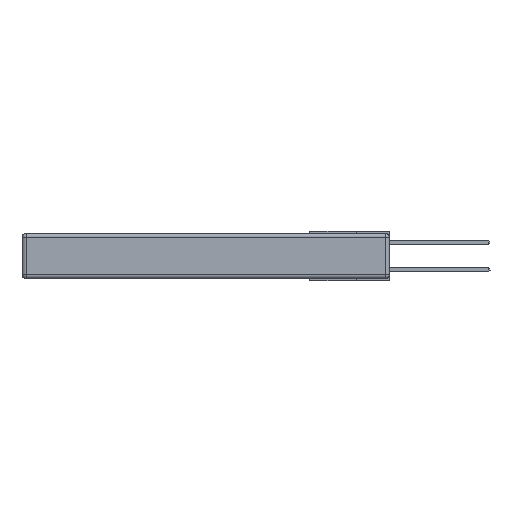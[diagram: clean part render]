
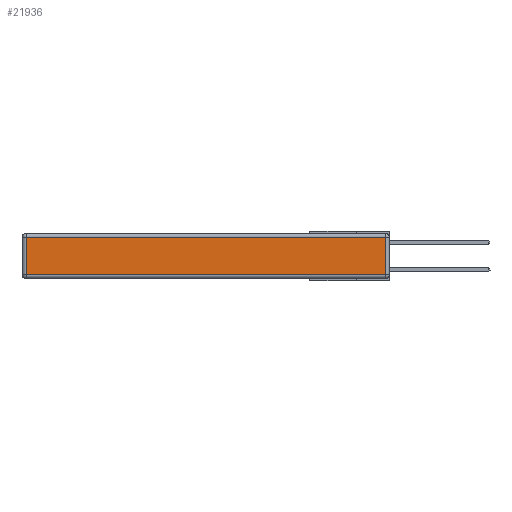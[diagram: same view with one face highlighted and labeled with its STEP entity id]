
A CAD part, left-side view. The second image highlights one B-rep face of the part: STEP entity #21936.
In plain terms, the highlighted planar face has unit normal (-1, 0, 0).
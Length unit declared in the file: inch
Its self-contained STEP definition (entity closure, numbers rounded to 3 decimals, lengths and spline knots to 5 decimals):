
#464 = LINE ( 'NONE', #14427, #15472 ) ;
#1362 = CARTESIAN_POINT ( 'NONE',  ( 0., 0.03, -0.343 ) ) ;
#1411 = EDGE_CURVE ( 'NONE', #14654, #3368, #2467, .T. ) ;
#1449 = VERTEX_POINT ( 'NONE', #4506 ) ;
#1462 = DIRECTION ( 'NONE',  ( 0., 0., 1. ) ) ;
#1732 = EDGE_CURVE ( 'NONE', #1449, #14654, #464, .T. ) ;
#2467 = LINE ( 'NONE', #4817, #17970 ) ;
#3368 = VERTEX_POINT ( 'NONE', #19218 ) ;
#3746 = CARTESIAN_POINT ( 'NONE',  ( 0., 0.03, -0.03 ) ) ;
#4506 = CARTESIAN_POINT ( 'NONE',  ( 0., 2.72, -0.03 ) ) ;
#4817 = CARTESIAN_POINT ( 'NONE',  ( 0., 0., -0.313 ) ) ;
#6805 = CARTESIAN_POINT ( 'NONE',  ( 0., 0., -0.343 ) ) ;
#7361 = ORIENTED_EDGE ( 'NONE', *, *, #1732, .T. ) ;
#7746 = EDGE_CURVE ( 'NONE', #3368, #11528, #14118, .T. ) ;
#9345 = DIRECTION ( 'NONE',  ( 0., 0., -1. ) ) ;
#9660 = CARTESIAN_POINT ( 'NONE',  ( 0., 2.75, -0.03 ) ) ;
#11528 = VERTEX_POINT ( 'NONE', #3746 ) ;
#11597 = DIRECTION ( 'NONE',  ( 0., 1., 0. ) ) ;
#12142 = DIRECTION ( 'NONE',  ( 0., 0., 1. ) ) ;
#14118 = LINE ( 'NONE', #1362, #16603 ) ;
#14427 = CARTESIAN_POINT ( 'NONE',  ( 0., 2.72, -0.343 ) ) ;
#14654 = VERTEX_POINT ( 'NONE', #17827 ) ;
#15472 = VECTOR ( 'NONE', #9345, 39.37008 ) ;
#15510 = ORIENTED_EDGE ( 'NONE', *, *, #18768, .T. ) ;
#15609 = ORIENTED_EDGE ( 'NONE', *, *, #1411, .T. ) ;
#15624 = ORIENTED_EDGE ( 'NONE', *, *, #7746, .T. ) ;
#16364 = EDGE_LOOP ( 'NONE', ( #15609, #15624, #15510, #7361 ) ) ;
#16603 = VECTOR ( 'NONE', #12142, 39.37008 ) ;
#17023 = VECTOR ( 'NONE', #11597, 39.37008 ) ;
#17142 = AXIS2_PLACEMENT_3D ( 'NONE', #6805, #17441, #1462 ) ;
#17441 = DIRECTION ( 'NONE',  ( -1., 0., 0. ) ) ;
#17827 = CARTESIAN_POINT ( 'NONE',  ( 0., 2.72, -0.313 ) ) ;
#17970 = VECTOR ( 'NONE', #18048, 39.37008 ) ;
#18048 = DIRECTION ( 'NONE',  ( 0., -1., 0. ) ) ;
#18768 = EDGE_CURVE ( 'NONE', #11528, #1449, #22479, .T. ) ;
#19218 = CARTESIAN_POINT ( 'NONE',  ( 0., 0.03, -0.313 ) ) ;
#20944 = PLANE ( 'NONE',  #17142 ) ;
#21936 = ADVANCED_FACE ( 'NONE', ( #22792 ), #20944, .T. ) ;
#22479 = LINE ( 'NONE', #9660, #17023 ) ;
#22792 = FACE_OUTER_BOUND ( 'NONE', #16364, .T. ) ;
